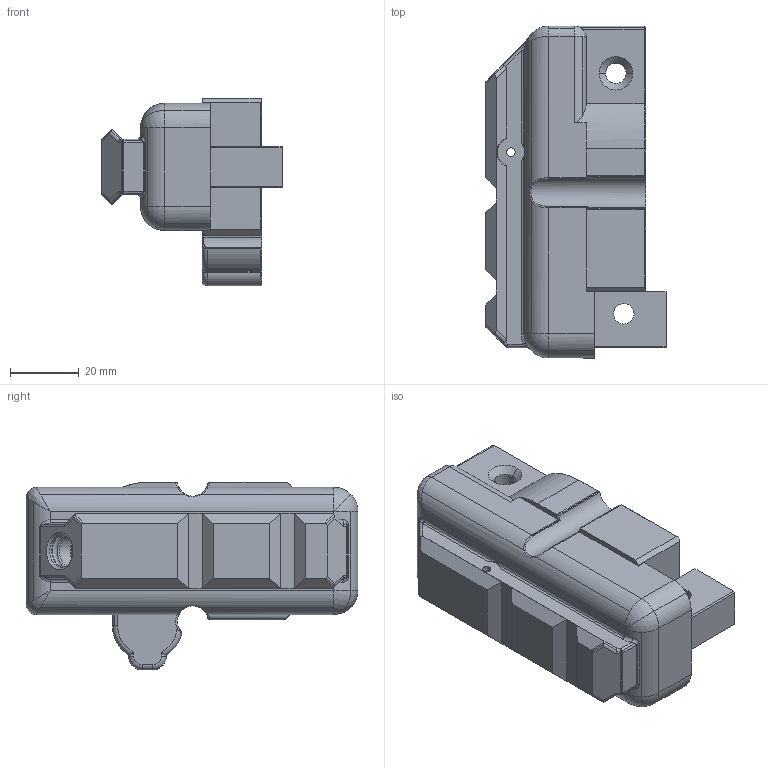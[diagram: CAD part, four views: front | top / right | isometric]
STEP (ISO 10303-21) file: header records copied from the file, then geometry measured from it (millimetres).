
FILE_DESCRIPTION(('STEP AP214'),'1');
FILE_NAME('Mod9 Hyd Buffer Endcap Fina;.stp','2020-09-28T22:43:32',(' '),(' '),'Spatial InterOp 3D',' ',' ');
FILE_SCHEMA(('AUTOMOTIVE_DESIGN { 1 0 10303 214 1 1 1 1 }'));
Length unit declared in the file: metre
Products named in the file (1): ASM Body
Bounding box: 52.54 x 96.84 x 54.82 mm (x, y, z)
Volume: 115118.3 mm3; surface area: 23716.7 mm2
Topology: 1 solids, 1 shells, 301 faces, 774 edges, 476 vertices
Faces by surface type: cylinder 141, plane 87, cone 28, torus 21, bspline 16, sphere 8
Entity records: 10194 total; most frequent: CARTESIAN_POINT 2780, DIRECTION 1606, ORIENTED_EDGE 1540, EDGE_CURVE 770, AXIS2_PLACEMENT_3D 617, VERTEX_POINT 476, LINE 372, VECTOR 372
